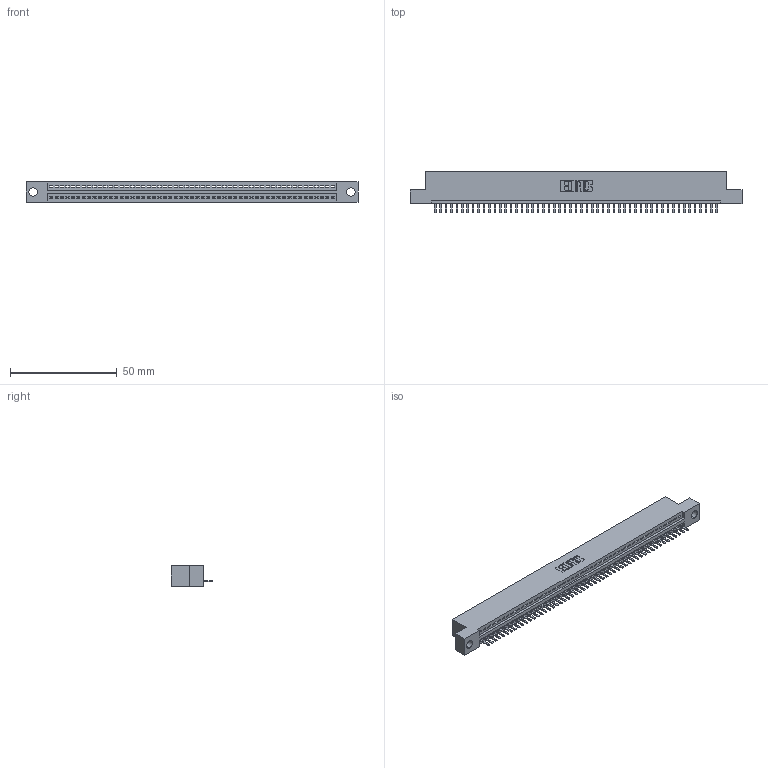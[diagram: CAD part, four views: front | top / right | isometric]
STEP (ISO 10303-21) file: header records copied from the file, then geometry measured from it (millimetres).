
FILE_DESCRIPTION (( 'STEP AP203' ), '1' );
FILE_NAME ('395-053-520-104.STEP', '2018-11-21T02:42:10', ( '' ), ( '' ), 'SwSTEP 2.0', 'SolidWorks 2016', '' );
FILE_SCHEMA (( 'CONFIG_CONTROL_DESIGN' ));
Length unit declared in the file: inch
Products named in the file (3): 345-292-001_345-293-120; 395-053-520-104; 345 Part_Flush Mounting Lugs - 0.156 Dia-TH
Assembly tree (54 placements, depth 2):
  395-053-520-104
    345 Part_Flush Mounting Lugs - 0.156 Dia-TH
    345-292-001_345-293-120  x53
Bounding box: 155.83 x 19.68 x 9.4 mm (x, y, z)
Volume: 14650.6 mm3; surface area: 18928.8 mm2
Topology: 54 solids, 54 shells, 3412 faces, 10093 edges, 6586 vertices
Faces by surface type: plane 2306, cylinder 1106
Entity records: 38525 total; most frequent: CARTESIAN_POINT 6691, ORIENTED_EDGE 6666, DIRECTION 5815, EDGE_CURVE 3333, LINE 2985, VECTOR 2985, VERTEX_POINT 2218, AXIS2_PLACEMENT_3D 1415
